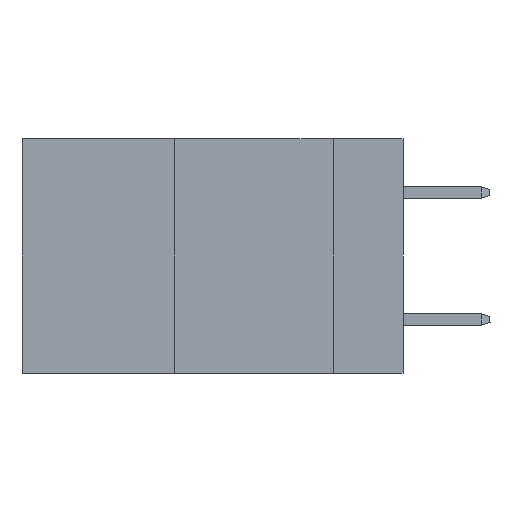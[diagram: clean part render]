
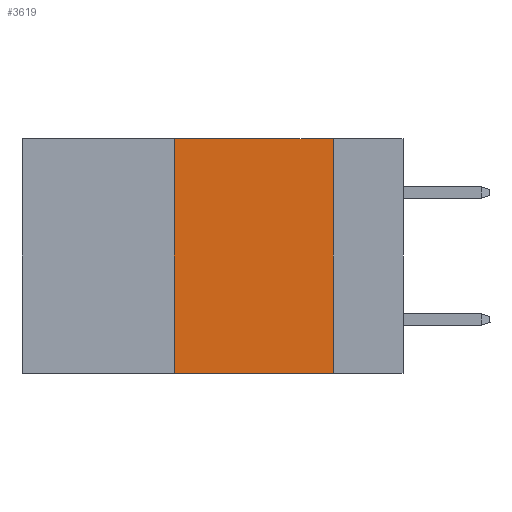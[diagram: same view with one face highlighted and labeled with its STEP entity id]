
A CAD part, left-side view. The second image highlights one B-rep face of the part: STEP entity #3619.
In plain terms, the highlighted planar face has unit normal (-1, 0, 0).
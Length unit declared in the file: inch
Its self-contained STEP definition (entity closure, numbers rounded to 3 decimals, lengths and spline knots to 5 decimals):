
#122 = LINE ( 'NONE', #4187, #13491 ) ;
#390 = EDGE_CURVE ( 'NONE', #6809, #4773, #122, .T. ) ;
#1348 = VECTOR ( 'NONE', #6137, 39.37008 ) ;
#1354 = AXIS2_PLACEMENT_3D ( 'NONE', #2496, #15141, #8135 ) ;
#1506 = DIRECTION ( 'NONE',  ( 0., 0., 1. ) ) ;
#2077 = ORIENTED_EDGE ( 'NONE', *, *, #6168, .F. ) ;
#2496 = CARTESIAN_POINT ( 'NONE',  ( 0., 0.6, 0. ) ) ;
#2778 = ORIENTED_EDGE ( 'NONE', *, *, #3752, .T. ) ;
#3420 = VECTOR ( 'NONE', #5633, 39.37008 ) ;
#3531 = DIRECTION ( 'NONE',  ( 0., 0., -1. ) ) ;
#3619 = ADVANCED_FACE ( 'NONE', ( #9510 ), #16173, .F. ) ;
#3752 = EDGE_CURVE ( 'NONE', #6809, #6602, #12479, .T. ) ;
#4187 = CARTESIAN_POINT ( 'NONE',  ( 0., 0.36, 0. ) ) ;
#4773 = VERTEX_POINT ( 'NONE', #14712 ) ;
#5152 = CARTESIAN_POINT ( 'NONE',  ( 0., 0.11, -0.37 ) ) ;
#5528 = VECTOR ( 'NONE', #3531, 39.37008 ) ;
#5633 = DIRECTION ( 'NONE',  ( 0., -1., 0. ) ) ;
#6137 = DIRECTION ( 'NONE',  ( 0., -1., 0. ) ) ;
#6145 = VERTEX_POINT ( 'NONE', #8638 ) ;
#6168 = EDGE_CURVE ( 'NONE', #4773, #6145, #13174, .T. ) ;
#6602 = VERTEX_POINT ( 'NONE', #5152 ) ;
#6809 = VERTEX_POINT ( 'NONE', #11677 ) ;
#8135 = DIRECTION ( 'NONE',  ( 0., 0., -1. ) ) ;
#8638 = CARTESIAN_POINT ( 'NONE',  ( 0., 0.11, 0. ) ) ;
#8869 = ORIENTED_EDGE ( 'NONE', *, *, #390, .F. ) ;
#9367 = EDGE_LOOP ( 'NONE', ( #17014, #2077, #8869, #2778 ) ) ;
#9510 = FACE_OUTER_BOUND ( 'NONE', #9367, .T. ) ;
#9527 = CARTESIAN_POINT ( 'NONE',  ( 0., 0.11, 0. ) ) ;
#10823 = LINE ( 'NONE', #9527, #5528 ) ;
#11620 = EDGE_CURVE ( 'NONE', #6145, #6602, #10823, .T. ) ;
#11677 = CARTESIAN_POINT ( 'NONE',  ( 0., 0.36, -0.37 ) ) ;
#12479 = LINE ( 'NONE', #13868, #3420 ) ;
#12976 = CARTESIAN_POINT ( 'NONE',  ( 0., 0.6, 0. ) ) ;
#13174 = LINE ( 'NONE', #12976, #1348 ) ;
#13491 = VECTOR ( 'NONE', #1506, 39.37008 ) ;
#13868 = CARTESIAN_POINT ( 'NONE',  ( 0., 0.6, -0.37 ) ) ;
#14712 = CARTESIAN_POINT ( 'NONE',  ( 0., 0.36, 0. ) ) ;
#15141 = DIRECTION ( 'NONE',  ( 1., 0., 0. ) ) ;
#16173 = PLANE ( 'NONE',  #1354 ) ;
#17014 = ORIENTED_EDGE ( 'NONE', *, *, #11620, .F. ) ;
